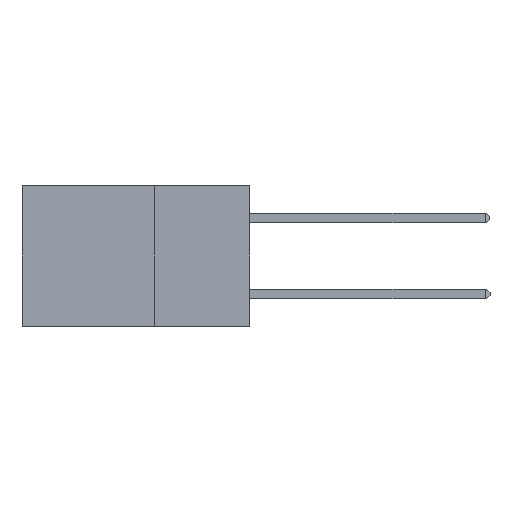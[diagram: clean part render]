
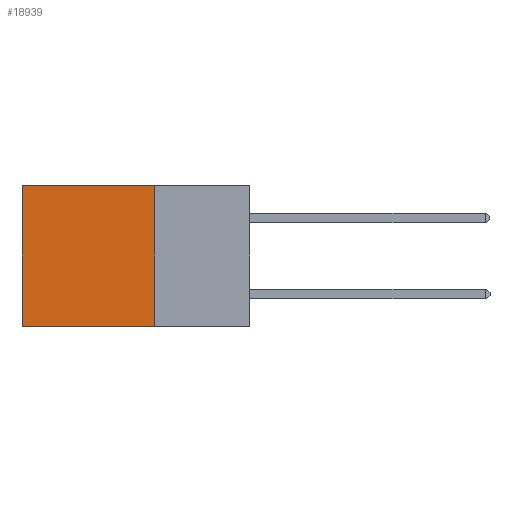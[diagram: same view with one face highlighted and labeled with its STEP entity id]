
A CAD part, left-side view. The second image highlights one B-rep face of the part: STEP entity #18939.
In plain terms, the highlighted planar face has unit normal (-1, 0, 0).
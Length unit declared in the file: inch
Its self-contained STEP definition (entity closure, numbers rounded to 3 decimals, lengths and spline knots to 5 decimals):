
#394 = ORIENTED_EDGE ( 'NONE', *, *, #1546, .T. ) ;
#481 = LINE ( 'NONE', #4589, #15331 ) ;
#1070 = LINE ( 'NONE', #10526, #11872 ) ;
#1416 = CARTESIAN_POINT ( 'NONE',  ( 0.2875, 0.25, 0. ) ) ;
#1509 = EDGE_CURVE ( 'NONE', #4942, #3755, #16277, .T. ) ;
#1546 = EDGE_CURVE ( 'NONE', #5220, #3755, #481, .T. ) ;
#2548 = AXIS2_PLACEMENT_3D ( 'NONE', #15682, #17194, #8287 ) ;
#2936 = DIRECTION ( 'NONE',  ( 0., 1., 0. ) ) ;
#3755 = VERTEX_POINT ( 'NONE', #8280 ) ;
#4497 = ORIENTED_EDGE ( 'NONE', *, *, #15894, .T. ) ;
#4589 = CARTESIAN_POINT ( 'NONE',  ( 0.2875, 0.6, 0. ) ) ;
#4750 = DIRECTION ( 'NONE',  ( 0., 0., -1. ) ) ;
#4942 = VERTEX_POINT ( 'NONE', #18226 ) ;
#5078 = DIRECTION ( 'NONE',  ( 0., 1., 0. ) ) ;
#5220 = VERTEX_POINT ( 'NONE', #18998 ) ;
#5386 = PLANE ( 'NONE',  #2548 ) ;
#5712 = CARTESIAN_POINT ( 'NONE',  ( 0.2875, 0.25, -0.37 ) ) ;
#6138 = EDGE_CURVE ( 'NONE', #11509, #4942, #1070, .T. ) ;
#7706 = VECTOR ( 'NONE', #2936, 39.37008 ) ;
#7827 = FACE_OUTER_BOUND ( 'NONE', #16848, .T. ) ;
#8280 = CARTESIAN_POINT ( 'NONE',  ( 0.2875, 0.6, -0.37 ) ) ;
#8287 = DIRECTION ( 'NONE',  ( 0., 0., -1. ) ) ;
#9973 = ORIENTED_EDGE ( 'NONE', *, *, #6138, .F. ) ;
#10526 = CARTESIAN_POINT ( 'NONE',  ( 0.2875, 0.25, 0. ) ) ;
#11509 = VERTEX_POINT ( 'NONE', #18688 ) ;
#11872 = VECTOR ( 'NONE', #15009, 39.37008 ) ;
#12231 = VECTOR ( 'NONE', #5078, 39.37008 ) ;
#15009 = DIRECTION ( 'NONE',  ( 0., 0., -1. ) ) ;
#15331 = VECTOR ( 'NONE', #4750, 39.37008 ) ;
#15581 = LINE ( 'NONE', #1416, #7706 ) ;
#15682 = CARTESIAN_POINT ( 'NONE',  ( 0.2875, 0.25, 0. ) ) ;
#15894 = EDGE_CURVE ( 'NONE', #11509, #5220, #15581, .T. ) ;
#16277 = LINE ( 'NONE', #5712, #12231 ) ;
#16848 = EDGE_LOOP ( 'NONE', ( #394, #18927, #9973, #4497 ) ) ;
#17194 = DIRECTION ( 'NONE',  ( 1., 0., 0. ) ) ;
#18226 = CARTESIAN_POINT ( 'NONE',  ( 0.2875, 0.25, -0.37 ) ) ;
#18688 = CARTESIAN_POINT ( 'NONE',  ( 0.2875, 0.25, 0. ) ) ;
#18927 = ORIENTED_EDGE ( 'NONE', *, *, #1509, .F. ) ;
#18939 = ADVANCED_FACE ( 'NONE', ( #7827 ), #5386, .F. ) ;
#18998 = CARTESIAN_POINT ( 'NONE',  ( 0.2875, 0.6, 0. ) ) ;
